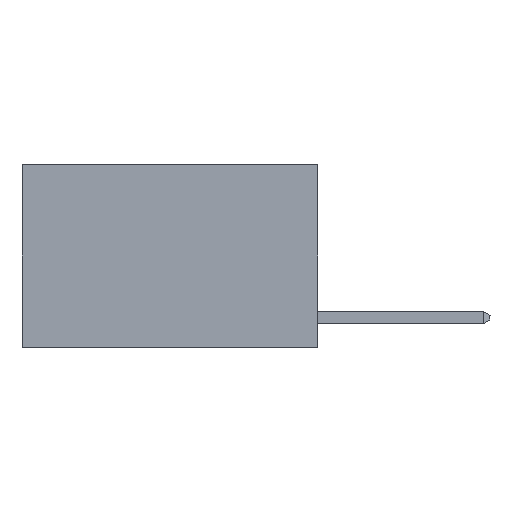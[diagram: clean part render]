
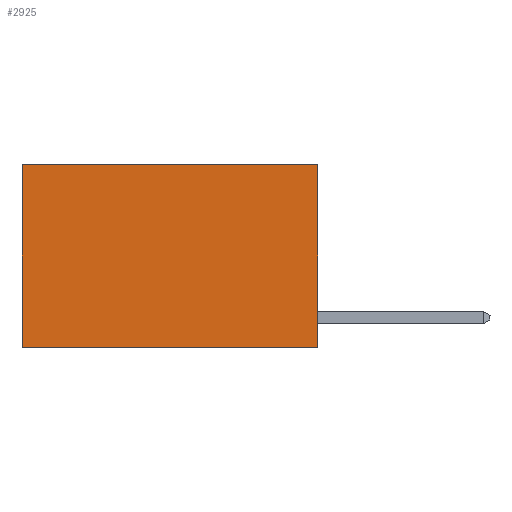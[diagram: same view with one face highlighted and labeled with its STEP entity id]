
A CAD part, left-side view. The second image highlights one B-rep face of the part: STEP entity #2925.
In plain terms, the highlighted planar face has unit normal (-1, 0, 0).
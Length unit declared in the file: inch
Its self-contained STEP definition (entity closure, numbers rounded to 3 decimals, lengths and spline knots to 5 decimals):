
#160 = LINE ( 'NONE', #23060, #867 ) ;
#256 = FACE_OUTER_BOUND ( 'NONE', #16011, .T. ) ;
#867 = VECTOR ( 'NONE', #7818, 39.37008 ) ;
#1208 = LINE ( 'NONE', #14873, #21276 ) ;
#1552 = AXIS2_PLACEMENT_3D ( 'NONE', #7793, #8040, #8165 ) ;
#2632 = LINE ( 'NONE', #18080, #22893 ) ;
#2925 = ADVANCED_FACE ( 'NONE', ( #256 ), #19738, .F. ) ;
#3023 = CARTESIAN_POINT ( 'NONE',  ( 0.2625, 0.6, 0. ) ) ;
#4790 = VERTEX_POINT ( 'NONE', #8946 ) ;
#7622 = VERTEX_POINT ( 'NONE', #3023 ) ;
#7793 = CARTESIAN_POINT ( 'NONE',  ( 0.2625, 0., 0. ) ) ;
#7818 = DIRECTION ( 'NONE',  ( 0., 0., -1. ) ) ;
#8040 = DIRECTION ( 'NONE',  ( 1., 0., 0. ) ) ;
#8165 = DIRECTION ( 'NONE',  ( 0., 0., -1. ) ) ;
#8946 = CARTESIAN_POINT ( 'NONE',  ( 0.2625, 0., -0.37 ) ) ;
#9240 = DIRECTION ( 'NONE',  ( 0., 0., -1. ) ) ;
#9396 = VERTEX_POINT ( 'NONE', #16529 ) ;
#10204 = DIRECTION ( 'NONE',  ( 0., 1., 0. ) ) ;
#10608 = ORIENTED_EDGE ( 'NONE', *, *, #13462, .T. ) ;
#12801 = VERTEX_POINT ( 'NONE', #24430 ) ;
#13462 = EDGE_CURVE ( 'NONE', #9396, #7622, #2632, .T. ) ;
#14699 = ORIENTED_EDGE ( 'NONE', *, *, #19508, .T. ) ;
#14873 = CARTESIAN_POINT ( 'NONE',  ( 0.2625, 0., 0. ) ) ;
#16011 = EDGE_LOOP ( 'NONE', ( #14699, #24139, #19021, #10608 ) ) ;
#16529 = CARTESIAN_POINT ( 'NONE',  ( 0.2625, 0., 0. ) ) ;
#16691 = EDGE_CURVE ( 'NONE', #9396, #4790, #1208, .T. ) ;
#17285 = CARTESIAN_POINT ( 'NONE',  ( 0.2625, 0., -0.37 ) ) ;
#18080 = CARTESIAN_POINT ( 'NONE',  ( 0.2625, 0., 0. ) ) ;
#18580 = VECTOR ( 'NONE', #10204, 39.37008 ) ;
#19021 = ORIENTED_EDGE ( 'NONE', *, *, #16691, .F. ) ;
#19198 = LINE ( 'NONE', #17285, #18580 ) ;
#19508 = EDGE_CURVE ( 'NONE', #7622, #12801, #160, .T. ) ;
#19738 = PLANE ( 'NONE',  #1552 ) ;
#19877 = DIRECTION ( 'NONE',  ( 0., 1., 0. ) ) ;
#21276 = VECTOR ( 'NONE', #9240, 39.37008 ) ;
#22893 = VECTOR ( 'NONE', #19877, 39.37008 ) ;
#22922 = EDGE_CURVE ( 'NONE', #4790, #12801, #19198, .T. ) ;
#23060 = CARTESIAN_POINT ( 'NONE',  ( 0.2625, 0.6, 0. ) ) ;
#24139 = ORIENTED_EDGE ( 'NONE', *, *, #22922, .F. ) ;
#24430 = CARTESIAN_POINT ( 'NONE',  ( 0.2625, 0.6, -0.37 ) ) ;
